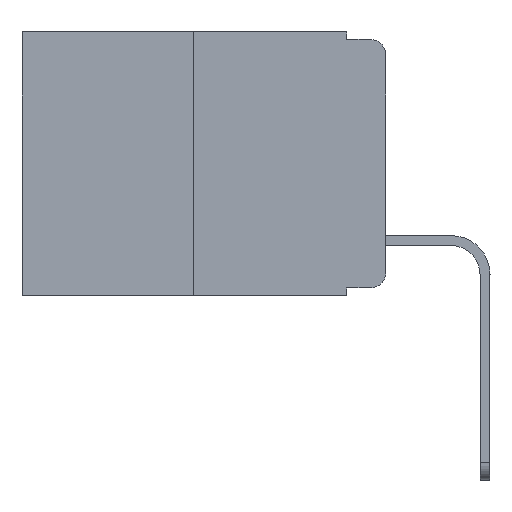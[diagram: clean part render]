
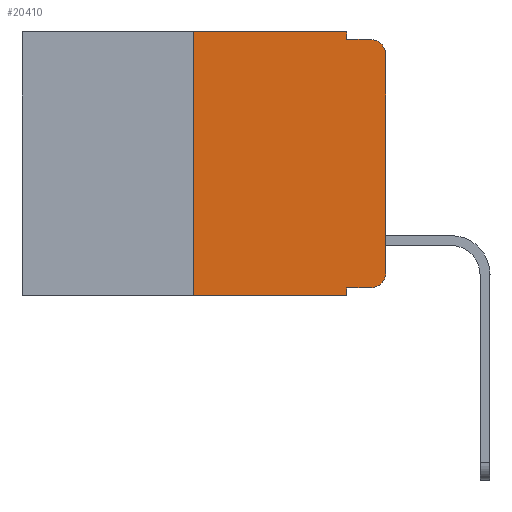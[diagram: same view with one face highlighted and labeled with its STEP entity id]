
A CAD part, left-side view. The second image highlights one B-rep face of the part: STEP entity #20410.
In plain terms, the highlighted planar face has unit normal (-1, 0, 0).
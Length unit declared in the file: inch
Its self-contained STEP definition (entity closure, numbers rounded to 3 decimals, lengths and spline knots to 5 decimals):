
#153 = VERTEX_POINT ( 'NONE', #3697 ) ;
#199 = DIRECTION ( 'NONE',  ( 0., 0., -1. ) ) ;
#622 = EDGE_LOOP ( 'NONE', ( #17620, #7944, #17373, #9868, #10380, #4248, #13278, #18927, #12045, #1362 ) ) ;
#1108 = CARTESIAN_POINT ( 'NONE',  ( 0., 0.051, 0. ) ) ;
#1362 = ORIENTED_EDGE ( 'NONE', *, *, #17674, .T. ) ;
#2101 = DIRECTION ( 'NONE',  ( 1., 0., 0. ) ) ;
#2420 = VECTOR ( 'NONE', #15312, 39.37008 ) ;
#2691 = VERTEX_POINT ( 'NONE', #6254 ) ;
#2825 = DIRECTION ( 'NONE',  ( 0., 0., -1. ) ) ;
#2991 = EDGE_CURVE ( 'NONE', #3901, #7465, #15468, .T. ) ;
#3172 = CARTESIAN_POINT ( 'NONE',  ( 0., 0.051, 0. ) ) ;
#3697 = CARTESIAN_POINT ( 'NONE',  ( 0., 0.051, -0.343 ) ) ;
#3717 = VERTEX_POINT ( 'NONE', #11731 ) ;
#3796 = PLANE ( 'NONE',  #3989 ) ;
#3832 = VECTOR ( 'NONE', #12635, 39.37008 ) ;
#3901 = VERTEX_POINT ( 'NONE', #14002 ) ;
#3989 = AXIS2_PLACEMENT_3D ( 'NONE', #12217, #2101, #13915 ) ;
#4078 = CARTESIAN_POINT ( 'NONE',  ( 0., 0., -0.313 ) ) ;
#4248 = ORIENTED_EDGE ( 'NONE', *, *, #16260, .F. ) ;
#4375 = EDGE_CURVE ( 'NONE', #15907, #7185, #8150, .T. ) ;
#4460 = CARTESIAN_POINT ( 'NONE',  ( 0., 0., -0.03 ) ) ;
#4619 = VECTOR ( 'NONE', #13405, 39.37008 ) ;
#5165 = CARTESIAN_POINT ( 'NONE',  ( 0., 0.25, 0. ) ) ;
#5199 = DIRECTION ( 'NONE',  ( 0., 0., 1. ) ) ;
#5266 = CARTESIAN_POINT ( 'NONE',  ( 0., 0.051, -0.01 ) ) ;
#5318 = CARTESIAN_POINT ( 'NONE',  ( 0., 0.25, -0.343 ) ) ;
#5515 = VECTOR ( 'NONE', #12305, 39.37008 ) ;
#5579 = CIRCLE ( 'NONE', #13010, 0.02 ) ;
#6254 = CARTESIAN_POINT ( 'NONE',  ( 0., 0.02, -0.01 ) ) ;
#6328 = VECTOR ( 'NONE', #13291, 39.37008 ) ;
#6597 = CARTESIAN_POINT ( 'NONE',  ( 0., 0.473, 0. ) ) ;
#6686 = VECTOR ( 'NONE', #16983, 39.37008 ) ;
#6948 = AXIS2_PLACEMENT_3D ( 'NONE', #9976, #15426, #199 ) ;
#7185 = VERTEX_POINT ( 'NONE', #4460 ) ;
#7327 = LINE ( 'NONE', #10538, #5515 ) ;
#7465 = VERTEX_POINT ( 'NONE', #5266 ) ;
#7944 = ORIENTED_EDGE ( 'NONE', *, *, #9315, .T. ) ;
#8090 = EDGE_CURVE ( 'NONE', #14822, #21431, #10359, .T. ) ;
#8150 = LINE ( 'NONE', #10369, #21356 ) ;
#8239 = CARTESIAN_POINT ( 'NONE',  ( 0., 0.051, -0.333 ) ) ;
#8354 = EDGE_CURVE ( 'NONE', #7465, #2691, #15365, .T. ) ;
#9100 = LINE ( 'NONE', #6597, #4619 ) ;
#9315 = EDGE_CURVE ( 'NONE', #7185, #2691, #10317, .T. ) ;
#9868 = ORIENTED_EDGE ( 'NONE', *, *, #2991, .F. ) ;
#9976 = CARTESIAN_POINT ( 'NONE',  ( 0., 0.02, -0.03 ) ) ;
#10317 = CIRCLE ( 'NONE', #6948, 0.02 ) ;
#10359 = LINE ( 'NONE', #8239, #13001 ) ;
#10369 = CARTESIAN_POINT ( 'NONE',  ( 0., 0., 0. ) ) ;
#10380 = ORIENTED_EDGE ( 'NONE', *, *, #11466, .F. ) ;
#10530 = CARTESIAN_POINT ( 'NONE',  ( 0., 0.051, -0.01 ) ) ;
#10538 = CARTESIAN_POINT ( 'NONE',  ( 0., 0.473, -0.343 ) ) ;
#10567 = LINE ( 'NONE', #3172, #6328 ) ;
#11466 = EDGE_CURVE ( 'NONE', #3717, #3901, #9100, .T. ) ;
#11644 = DIRECTION ( 'NONE',  ( 0., -1., 0. ) ) ;
#11731 = CARTESIAN_POINT ( 'NONE',  ( 0., 0.25, 0. ) ) ;
#12045 = ORIENTED_EDGE ( 'NONE', *, *, #8090, .T. ) ;
#12217 = CARTESIAN_POINT ( 'NONE',  ( 0., 0.473, 0. ) ) ;
#12305 = DIRECTION ( 'NONE',  ( 0., -1., 0. ) ) ;
#12635 = DIRECTION ( 'NONE',  ( 0., 0., -1. ) ) ;
#13001 = VECTOR ( 'NONE', #11644, 39.37008 ) ;
#13010 = AXIS2_PLACEMENT_3D ( 'NONE', #19553, #15975, #2825 ) ;
#13278 = ORIENTED_EDGE ( 'NONE', *, *, #18799, .T. ) ;
#13291 = DIRECTION ( 'NONE',  ( 0., 0., -1. ) ) ;
#13405 = DIRECTION ( 'NONE',  ( 0., -1., 0. ) ) ;
#13845 = EDGE_CURVE ( 'NONE', #14822, #153, #10567, .T. ) ;
#13915 = DIRECTION ( 'NONE',  ( 0., 0., -1. ) ) ;
#14002 = CARTESIAN_POINT ( 'NONE',  ( 0., 0.051, 0. ) ) ;
#14738 = CARTESIAN_POINT ( 'NONE',  ( 0., 0.051, -0.333 ) ) ;
#14822 = VERTEX_POINT ( 'NONE', #14738 ) ;
#15140 = LINE ( 'NONE', #5165, #6686 ) ;
#15312 = DIRECTION ( 'NONE',  ( 0., -1., 0. ) ) ;
#15365 = LINE ( 'NONE', #10530, #2420 ) ;
#15426 = DIRECTION ( 'NONE',  ( -1., 0., 0. ) ) ;
#15468 = LINE ( 'NONE', #1108, #3832 ) ;
#15717 = FACE_OUTER_BOUND ( 'NONE', #622, .T. ) ;
#15907 = VERTEX_POINT ( 'NONE', #4078 ) ;
#15975 = DIRECTION ( 'NONE',  ( -1., 0., 0. ) ) ;
#16260 = EDGE_CURVE ( 'NONE', #21731, #3717, #15140, .T. ) ;
#16337 = CARTESIAN_POINT ( 'NONE',  ( 0., 0.02, -0.333 ) ) ;
#16983 = DIRECTION ( 'NONE',  ( 0., 0., 1. ) ) ;
#17373 = ORIENTED_EDGE ( 'NONE', *, *, #8354, .F. ) ;
#17620 = ORIENTED_EDGE ( 'NONE', *, *, #4375, .T. ) ;
#17674 = EDGE_CURVE ( 'NONE', #21431, #15907, #5579, .T. ) ;
#18799 = EDGE_CURVE ( 'NONE', #21731, #153, #7327, .T. ) ;
#18927 = ORIENTED_EDGE ( 'NONE', *, *, #13845, .F. ) ;
#19553 = CARTESIAN_POINT ( 'NONE',  ( 0., 0.02, -0.313 ) ) ;
#20410 = ADVANCED_FACE ( 'NONE', ( #15717 ), #3796, .F. ) ;
#21356 = VECTOR ( 'NONE', #5199, 39.37008 ) ;
#21431 = VERTEX_POINT ( 'NONE', #16337 ) ;
#21731 = VERTEX_POINT ( 'NONE', #5318 ) ;
